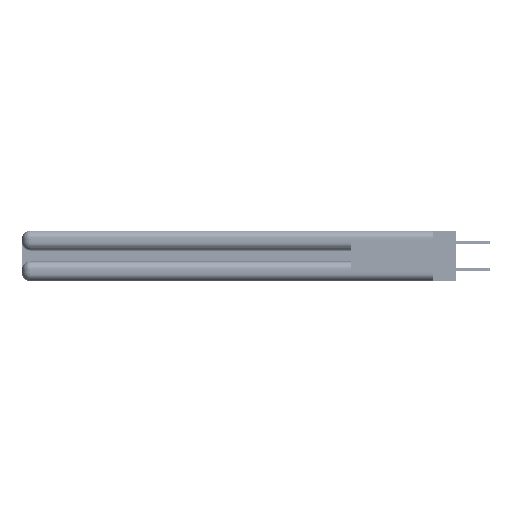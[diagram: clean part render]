
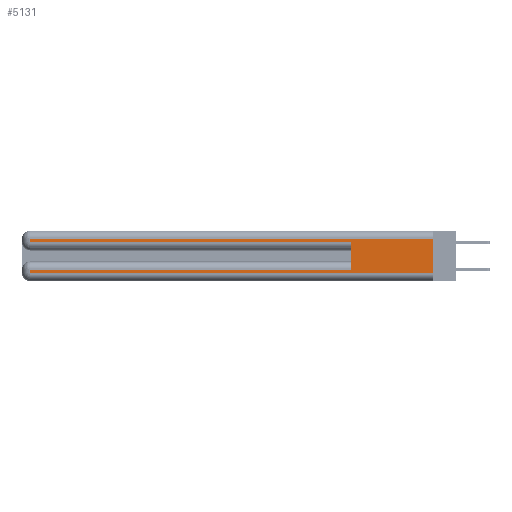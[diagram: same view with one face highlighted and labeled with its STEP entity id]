
A CAD part, left-side view. The second image highlights one B-rep face of the part: STEP entity #5131.
In plain terms, the highlighted planar face has unit normal (-1, 0, 0).
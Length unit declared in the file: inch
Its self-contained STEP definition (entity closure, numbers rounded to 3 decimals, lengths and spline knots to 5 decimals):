
#856 = PLANE ( 'NONE',  #28398 ) ;
#1351 = ORIENTED_EDGE ( 'NONE', *, *, #46105, .T. ) ;
#1523 = VECTOR ( 'NONE', #16394, 39.37008 ) ;
#2370 = CARTESIAN_POINT ( 'NONE',  ( 0., 0., 0.37 ) ) ;
#3101 = EDGE_CURVE ( 'NONE', #22704, #16811, #14511, .T. ) ;
#4441 = DIRECTION ( 'NONE',  ( 0., 0., -1. ) ) ;
#5131 = ADVANCED_FACE ( 'NONE', ( #8063 ), #856, .F. ) ;
#6632 = VECTOR ( 'NONE', #40090, 39.37008 ) ;
#7346 = VECTOR ( 'NONE', #14424, 39.37008 ) ;
#7710 = DIRECTION ( 'NONE',  ( 0., -1., 0. ) ) ;
#7848 = CARTESIAN_POINT ( 'NONE',  ( 0., 0., 0.085 ) ) ;
#8063 = FACE_OUTER_BOUND ( 'NONE', #24419, .T. ) ;
#8751 = CARTESIAN_POINT ( 'NONE',  ( 0., 0., 0.37 ) ) ;
#8857 = EDGE_CURVE ( 'NONE', #30991, #27171, #46052, .T. ) ;
#11589 = ORIENTED_EDGE ( 'NONE', *, *, #51109, .T. ) ;
#12908 = CARTESIAN_POINT ( 'NONE',  ( 0., 2.94, 0.085 ) ) ;
#13360 = ORIENTED_EDGE ( 'NONE', *, *, #36163, .F. ) ;
#14424 = DIRECTION ( 'NONE',  ( 0., 0., -1. ) ) ;
#14511 = LINE ( 'NONE', #45026, #21340 ) ;
#15942 = VECTOR ( 'NONE', #4441, 39.37008 ) ;
#16394 = DIRECTION ( 'NONE',  ( 0., 0., 1. ) ) ;
#16811 = VERTEX_POINT ( 'NONE', #50384 ) ;
#17478 = ORIENTED_EDGE ( 'NONE', *, *, #8857, .F. ) ;
#19749 = ORIENTED_EDGE ( 'NONE', *, *, #51178, .T. ) ;
#19912 = CARTESIAN_POINT ( 'NONE',  ( 0., 0.6, 0.145 ) ) ;
#20237 = ORIENTED_EDGE ( 'NONE', *, *, #25516, .T. ) ;
#20409 = VERTEX_POINT ( 'NONE', #32522 ) ;
#21141 = CARTESIAN_POINT ( 'NONE',  ( 0., 0.6, 0.085 ) ) ;
#21340 = VECTOR ( 'NONE', #35027, 39.37008 ) ;
#21886 = VERTEX_POINT ( 'NONE', #12908 ) ;
#22704 = VERTEX_POINT ( 'NONE', #34445 ) ;
#24044 = LINE ( 'NONE', #36357, #15942 ) ;
#24419 = EDGE_LOOP ( 'NONE', ( #13360, #45345, #11589, #20237, #17478, #19749, #44902, #1351 ) ) ;
#24800 = LINE ( 'NONE', #2370, #7346 ) ;
#25516 = EDGE_CURVE ( 'NONE', #20409, #27171, #36471, .T. ) ;
#25549 = CARTESIAN_POINT ( 'NONE',  ( 0., 0., 0.285 ) ) ;
#26194 = CARTESIAN_POINT ( 'NONE',  ( 0., 0., 0.06 ) ) ;
#26285 = VERTEX_POINT ( 'NONE', #26194 ) ;
#27171 = VERTEX_POINT ( 'NONE', #39765 ) ;
#28398 = AXIS2_PLACEMENT_3D ( 'NONE', #8751, #33480, #29765 ) ;
#28675 = VERTEX_POINT ( 'NONE', #44872 ) ;
#29135 = LINE ( 'NONE', #7848, #33572 ) ;
#29408 = DIRECTION ( 'NONE',  ( 0., -1., 0. ) ) ;
#29765 = DIRECTION ( 'NONE',  ( 0., 0., -1. ) ) ;
#30991 = VERTEX_POINT ( 'NONE', #21141 ) ;
#32522 = CARTESIAN_POINT ( 'NONE',  ( 0., 2.94, 0.285 ) ) ;
#33480 = DIRECTION ( 'NONE',  ( 1., 0., 0. ) ) ;
#33572 = VECTOR ( 'NONE', #44313, 39.37008 ) ;
#34418 = VECTOR ( 'NONE', #7710, 39.37008 ) ;
#34445 = CARTESIAN_POINT ( 'NONE',  ( 0., 0., 0.31 ) ) ;
#34857 = LINE ( 'NONE', #36248, #6632 ) ;
#35027 = DIRECTION ( 'NONE',  ( 0., 1., 0. ) ) ;
#36163 = EDGE_CURVE ( 'NONE', #22704, #26285, #24800, .T. ) ;
#36248 = CARTESIAN_POINT ( 'NONE',  ( 0., 2.94, 0.37 ) ) ;
#36357 = CARTESIAN_POINT ( 'NONE',  ( 0., 2.94, 0.37 ) ) ;
#36471 = LINE ( 'NONE', #25549, #44617 ) ;
#37855 = EDGE_CURVE ( 'NONE', #21886, #28675, #24044, .T. ) ;
#39765 = CARTESIAN_POINT ( 'NONE',  ( 0., 0.6, 0.285 ) ) ;
#40090 = DIRECTION ( 'NONE',  ( 0., 0., -1. ) ) ;
#43668 = CARTESIAN_POINT ( 'NONE',  ( 0., 0., 0.06 ) ) ;
#44313 = DIRECTION ( 'NONE',  ( 0., 1., 0. ) ) ;
#44617 = VECTOR ( 'NONE', #29408, 39.37008 ) ;
#44872 = CARTESIAN_POINT ( 'NONE',  ( 0., 2.94, 0.06 ) ) ;
#44902 = ORIENTED_EDGE ( 'NONE', *, *, #37855, .T. ) ;
#45026 = CARTESIAN_POINT ( 'NONE',  ( 0., 0., 0.31 ) ) ;
#45345 = ORIENTED_EDGE ( 'NONE', *, *, #3101, .T. ) ;
#46052 = LINE ( 'NONE', #19912, #1523 ) ;
#46105 = EDGE_CURVE ( 'NONE', #28675, #26285, #51315, .T. ) ;
#50384 = CARTESIAN_POINT ( 'NONE',  ( 0., 2.94, 0.31 ) ) ;
#51109 = EDGE_CURVE ( 'NONE', #16811, #20409, #34857, .T. ) ;
#51178 = EDGE_CURVE ( 'NONE', #30991, #21886, #29135, .T. ) ;
#51315 = LINE ( 'NONE', #43668, #34418 ) ;
